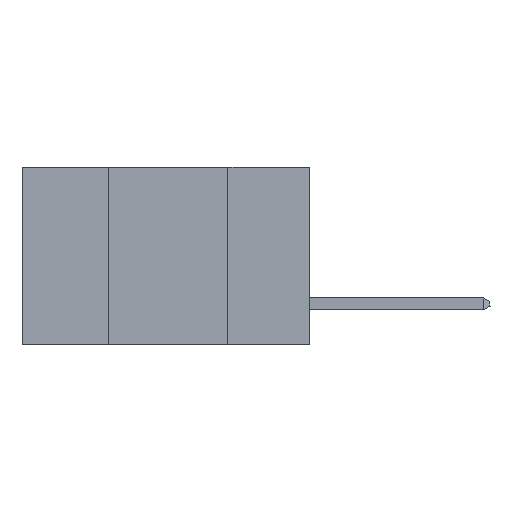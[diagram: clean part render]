
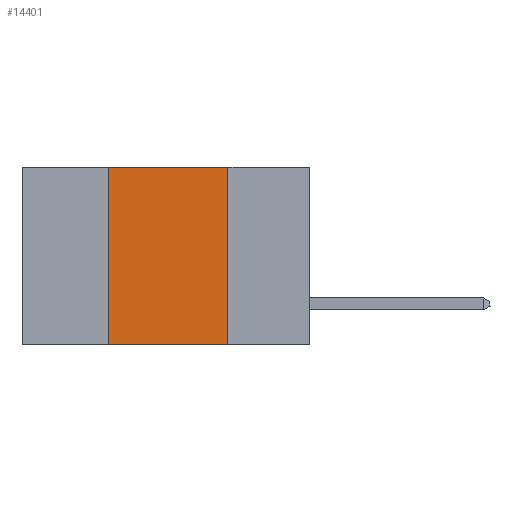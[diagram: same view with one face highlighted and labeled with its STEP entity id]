
A CAD part, left-side view. The second image highlights one B-rep face of the part: STEP entity #14401.
In plain terms, the highlighted planar face has unit normal (-1, 0, 0).
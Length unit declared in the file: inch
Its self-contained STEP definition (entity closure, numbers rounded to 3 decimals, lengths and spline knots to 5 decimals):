
#261 = DIRECTION ( 'NONE',  ( 1., 0., 0. ) ) ;
#1047 = VERTEX_POINT ( 'NONE', #11697 ) ;
#1773 = EDGE_CURVE ( 'NONE', #5750, #23877, #25952, .T. ) ;
#1843 = FACE_OUTER_BOUND ( 'NONE', #4754, .T. ) ;
#2840 = ORIENTED_EDGE ( 'NONE', *, *, #2914, .F. ) ;
#2914 = EDGE_CURVE ( 'NONE', #1047, #7184, #23967, .T. ) ;
#4754 = EDGE_LOOP ( 'NONE', ( #23311, #29917, #2840, #17374 ) ) ;
#4943 = PLANE ( 'NONE',  #27652 ) ;
#5389 = CARTESIAN_POINT ( 'NONE',  ( 0., 0.17, -0.37 ) ) ;
#5750 = VERTEX_POINT ( 'NONE', #10074 ) ;
#7184 = VERTEX_POINT ( 'NONE', #30282 ) ;
#8614 = VECTOR ( 'NONE', #17465, 39.37008 ) ;
#10074 = CARTESIAN_POINT ( 'NONE',  ( 0., 0.17, 0. ) ) ;
#11166 = VECTOR ( 'NONE', #11595, 39.37008 ) ;
#11595 = DIRECTION ( 'NONE',  ( 0., -1., 0. ) ) ;
#11697 = CARTESIAN_POINT ( 'NONE',  ( 0., 0.42, -0.37 ) ) ;
#12110 = DIRECTION ( 'NONE',  ( 0., 0., -1. ) ) ;
#13519 = CARTESIAN_POINT ( 'NONE',  ( 0., 0.6, -0.37 ) ) ;
#14401 = ADVANCED_FACE ( 'NONE', ( #1843 ), #4943, .F. ) ;
#15959 = LINE ( 'NONE', #13519, #16682 ) ;
#16682 = VECTOR ( 'NONE', #27852, 39.37008 ) ;
#17374 = ORIENTED_EDGE ( 'NONE', *, *, #29334, .T. ) ;
#17465 = DIRECTION ( 'NONE',  ( 0., 0., -1. ) ) ;
#18690 = CARTESIAN_POINT ( 'NONE',  ( 0., 0.6, 0. ) ) ;
#19561 = VECTOR ( 'NONE', #28702, 39.37008 ) ;
#23311 = ORIENTED_EDGE ( 'NONE', *, *, #1773, .F. ) ;
#23877 = VERTEX_POINT ( 'NONE', #5389 ) ;
#23955 = CARTESIAN_POINT ( 'NONE',  ( 0., 0.42, 0. ) ) ;
#23967 = LINE ( 'NONE', #23955, #19561 ) ;
#24114 = LINE ( 'NONE', #18690, #11166 ) ;
#24788 = CARTESIAN_POINT ( 'NONE',  ( 0., 0.17, 0. ) ) ;
#25910 = CARTESIAN_POINT ( 'NONE',  ( 0., 0.6, 0. ) ) ;
#25952 = LINE ( 'NONE', #24788, #8614 ) ;
#26172 = EDGE_CURVE ( 'NONE', #7184, #5750, #24114, .T. ) ;
#27652 = AXIS2_PLACEMENT_3D ( 'NONE', #25910, #261, #12110 ) ;
#27852 = DIRECTION ( 'NONE',  ( 0., -1., 0. ) ) ;
#28702 = DIRECTION ( 'NONE',  ( 0., 0., 1. ) ) ;
#29334 = EDGE_CURVE ( 'NONE', #1047, #23877, #15959, .T. ) ;
#29917 = ORIENTED_EDGE ( 'NONE', *, *, #26172, .F. ) ;
#30282 = CARTESIAN_POINT ( 'NONE',  ( 0., 0.42, 0. ) ) ;
